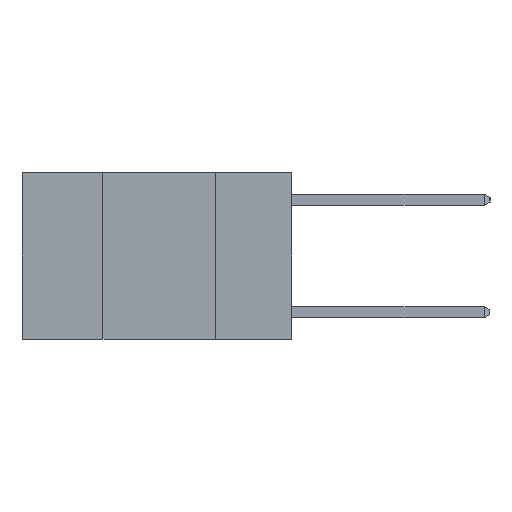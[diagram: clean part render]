
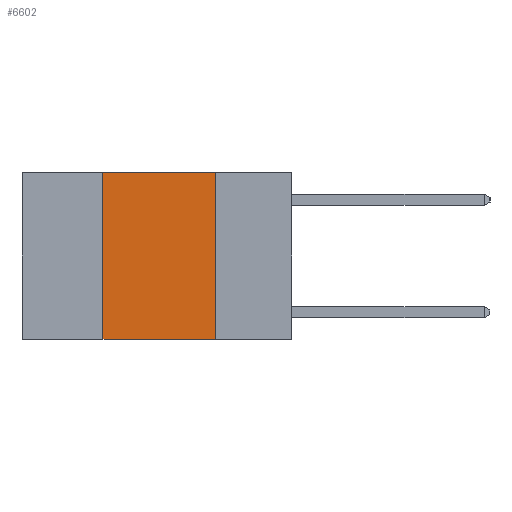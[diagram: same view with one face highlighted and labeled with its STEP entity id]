
A CAD part, left-side view. The second image highlights one B-rep face of the part: STEP entity #6602.
In plain terms, the highlighted planar face has unit normal (-1, 0, 0).
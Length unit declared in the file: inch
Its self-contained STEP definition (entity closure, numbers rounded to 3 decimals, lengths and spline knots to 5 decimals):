
#135 = ORIENTED_EDGE ( 'NONE', *, *, #1240, .F. ) ;
#154 = ORIENTED_EDGE ( 'NONE', *, *, #7820, .F. ) ;
#162 = ORIENTED_EDGE ( 'NONE', *, *, #878, .F. ) ;
#192 = ORIENTED_EDGE ( 'NONE', *, *, #5215, .T. ) ;
#268 = VECTOR ( 'NONE', #3888, 39.37008 ) ;
#622 = VERTEX_POINT ( 'NONE', #6860 ) ;
#797 = CARTESIAN_POINT ( 'NONE',  ( 0., 0.17, -0.37 ) ) ;
#878 = EDGE_CURVE ( 'NONE', #7952, #3373, #6168, .T. ) ;
#1143 = DIRECTION ( 'NONE',  ( 0., 0., -1. ) ) ;
#1156 = DIRECTION ( 'NONE',  ( 1., 0., 0. ) ) ;
#1169 = CARTESIAN_POINT ( 'NONE',  ( 0., 0.6, 0. ) ) ;
#1211 = DIRECTION ( 'NONE',  ( 0., -1., 0. ) ) ;
#1228 = CARTESIAN_POINT ( 'NONE',  ( 0., 0.6, -0.37 ) ) ;
#1240 = EDGE_CURVE ( 'NONE', #622, #6726, #5645, .T. ) ;
#1308 = PLANE ( 'NONE',  #8396 ) ;
#2409 = EDGE_LOOP ( 'NONE', ( #135, #154, #162, #192 ) ) ;
#2478 = VECTOR ( 'NONE', #7414, 39.37008 ) ;
#2489 = LINE ( 'NONE', #7470, #2478 ) ;
#3373 = VERTEX_POINT ( 'NONE', #4617 ) ;
#3888 = DIRECTION ( 'NONE',  ( 0., 0., -1. ) ) ;
#4028 = VECTOR ( 'NONE', #1211, 39.37008 ) ;
#4054 = CARTESIAN_POINT ( 'NONE',  ( 0., 0.17, 0. ) ) ;
#4617 = CARTESIAN_POINT ( 'NONE',  ( 0., 0.42, 0. ) ) ;
#4759 = LINE ( 'NONE', #1228, #4028 ) ;
#5178 = DIRECTION ( 'NONE',  ( 0., 0., 1. ) ) ;
#5215 = EDGE_CURVE ( 'NONE', #7952, #6726, #4759, .T. ) ;
#5645 = LINE ( 'NONE', #4054, #268 ) ;
#6098 = FACE_OUTER_BOUND ( 'NONE', #2409, .T. ) ;
#6168 = LINE ( 'NONE', #6471, #6189 ) ;
#6189 = VECTOR ( 'NONE', #5178, 39.37008 ) ;
#6471 = CARTESIAN_POINT ( 'NONE',  ( 0., 0.42, 0. ) ) ;
#6602 = ADVANCED_FACE ( 'NONE', ( #6098 ), #1308, .F. ) ;
#6726 = VERTEX_POINT ( 'NONE', #797 ) ;
#6763 = CARTESIAN_POINT ( 'NONE',  ( 0., 0.42, -0.37 ) ) ;
#6860 = CARTESIAN_POINT ( 'NONE',  ( 0., 0.17, 0. ) ) ;
#7414 = DIRECTION ( 'NONE',  ( 0., -1., 0. ) ) ;
#7470 = CARTESIAN_POINT ( 'NONE',  ( 0., 0.6, 0. ) ) ;
#7820 = EDGE_CURVE ( 'NONE', #3373, #622, #2489, .T. ) ;
#7952 = VERTEX_POINT ( 'NONE', #6763 ) ;
#8396 = AXIS2_PLACEMENT_3D ( 'NONE', #1169, #1156, #1143 ) ;
